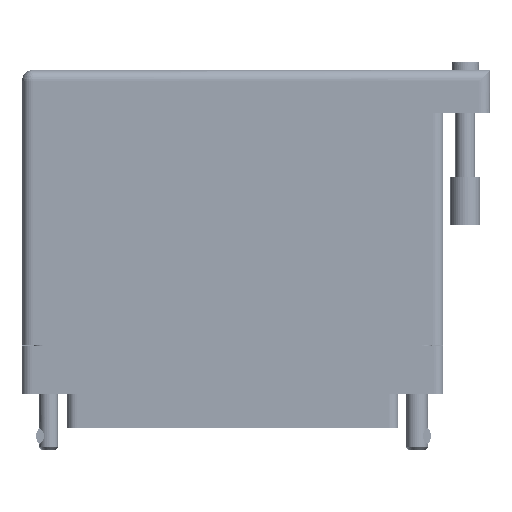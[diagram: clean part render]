
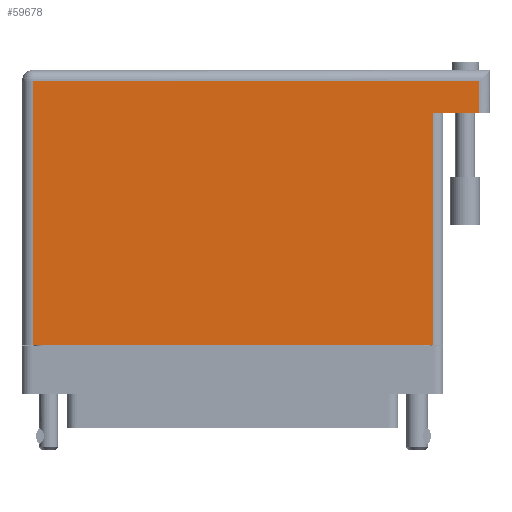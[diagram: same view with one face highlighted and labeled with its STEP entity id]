
A CAD part, front view. The second image highlights one B-rep face of the part: STEP entity #59678.
In plain terms, the highlighted face is planar.
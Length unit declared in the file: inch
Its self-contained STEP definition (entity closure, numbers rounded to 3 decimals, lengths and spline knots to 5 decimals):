
#2346 = VERTEX_POINT ( 'NONE', #41374 ) ;
#4002 = VERTEX_POINT ( 'NONE', #55672 ) ;
#6227 = VECTOR ( 'NONE', #31711, 39.37008 ) ;
#8118 = VECTOR ( 'NONE', #15122, 39.37008 ) ;
#11068 = DIRECTION ( 'NONE',  ( 1., 0., 0. ) ) ;
#11169 = ORIENTED_EDGE ( 'NONE', *, *, #30447, .T. ) ;
#11657 = VERTEX_POINT ( 'NONE', #37363 ) ;
#13140 = LINE ( 'NONE', #33270, #81086 ) ;
#13626 = DIRECTION ( 'NONE',  ( -1., 0., 0. ) ) ;
#13994 = AXIS2_PLACEMENT_3D ( 'NONE', #78137, #39373, #13626 ) ;
#14166 = VECTOR ( 'NONE', #11068, 39.37008 ) ;
#15122 = DIRECTION ( 'NONE',  ( 0., 1., 0. ) ) ;
#15186 = CARTESIAN_POINT ( 'NONE',  ( -1.289, 1.605, 0.617 ) ) ;
#16005 = VECTOR ( 'NONE', #52977, 39.37008 ) ;
#21280 = EDGE_LOOP ( 'NONE', ( #11169, #50142, #64191, #37061, #25725, #52375 ) ) ;
#22644 = CARTESIAN_POINT ( 'NONE',  ( 1.659, 1.395, 0.617 ) ) ;
#25725 = ORIENTED_EDGE ( 'NONE', *, *, #51336, .T. ) ;
#28450 = CARTESIAN_POINT ( 'NONE',  ( 1.289, 1.395, 0.617 ) ) ;
#30345 = LINE ( 'NONE', #28450, #8118 ) ;
#30447 = EDGE_CURVE ( 'NONE', #11657, #2346, #45523, .T. ) ;
#31711 = DIRECTION ( 'NONE',  ( 0., 1., 0. ) ) ;
#32877 = PLANE ( 'NONE',  #13994 ) ;
#33270 = CARTESIAN_POINT ( 'NONE',  ( -1.359, 1.605, 0.617 ) ) ;
#34186 = VERTEX_POINT ( 'NONE', #40821 ) ;
#37061 = ORIENTED_EDGE ( 'NONE', *, *, #79028, .T. ) ;
#37363 = CARTESIAN_POINT ( 'NONE',  ( -1.289, -0.1, 0.617 ) ) ;
#39163 = VECTOR ( 'NONE', #74429, 39.37008 ) ;
#39373 = DIRECTION ( 'NONE',  ( 0., 0., -1. ) ) ;
#40787 = FACE_OUTER_BOUND ( 'NONE', #21280, .T. ) ;
#40821 = CARTESIAN_POINT ( 'NONE',  ( 1.589, 1.395, 0.617 ) ) ;
#41374 = CARTESIAN_POINT ( 'NONE',  ( 1.289, -0.1, 0.617 ) ) ;
#45523 = LINE ( 'NONE', #76957, #14166 ) ;
#46578 = DIRECTION ( 'NONE',  ( -1., 0., 0. ) ) ;
#49362 = CARTESIAN_POINT ( 'NONE',  ( 1.589, 1.675, 0.617 ) ) ;
#50142 = ORIENTED_EDGE ( 'NONE', *, *, #68621, .T. ) ;
#50264 = EDGE_CURVE ( 'NONE', #34186, #4002, #53483, .T. ) ;
#50428 = LINE ( 'NONE', #79794, #16005 ) ;
#51294 = CARTESIAN_POINT ( 'NONE',  ( 1.589, 1.605, 0.617 ) ) ;
#51336 = EDGE_CURVE ( 'NONE', #80308, #72025, #13140, .T. ) ;
#52375 = ORIENTED_EDGE ( 'NONE', *, *, #75741, .T. ) ;
#52977 = DIRECTION ( 'NONE',  ( 0., -1., 0. ) ) ;
#53483 = LINE ( 'NONE', #22644, #39163 ) ;
#55672 = CARTESIAN_POINT ( 'NONE',  ( 1.289, 1.395, 0.617 ) ) ;
#59678 = ADVANCED_FACE ( 'NONE', ( #40787 ), #32877, .F. ) ;
#64191 = ORIENTED_EDGE ( 'NONE', *, *, #50264, .F. ) ;
#68621 = EDGE_CURVE ( 'NONE', #2346, #4002, #30345, .T. ) ;
#72025 = VERTEX_POINT ( 'NONE', #15186 ) ;
#74429 = DIRECTION ( 'NONE',  ( -1., 0., 0. ) ) ;
#75741 = EDGE_CURVE ( 'NONE', #72025, #11657, #50428, .T. ) ;
#76957 = CARTESIAN_POINT ( 'NONE',  ( -1.359, -0.1, 0.617 ) ) ;
#78088 = LINE ( 'NONE', #49362, #6227 ) ;
#78137 = CARTESIAN_POINT ( 'NONE',  ( -1.359, 1.675, 0.617 ) ) ;
#79028 = EDGE_CURVE ( 'NONE', #34186, #80308, #78088, .T. ) ;
#79794 = CARTESIAN_POINT ( 'NONE',  ( -1.289, -0.1, 0.617 ) ) ;
#80308 = VERTEX_POINT ( 'NONE', #51294 ) ;
#81086 = VECTOR ( 'NONE', #46578, 39.37008 ) ;
